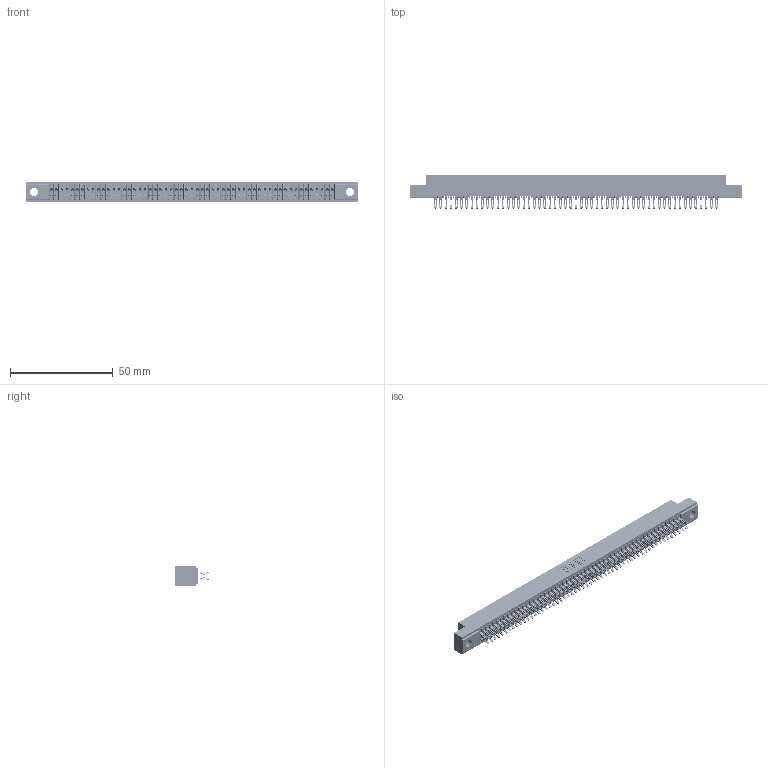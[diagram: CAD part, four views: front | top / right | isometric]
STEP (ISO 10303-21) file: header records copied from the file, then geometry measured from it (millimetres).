
FILE_DESCRIPTION (( 'STEP AP203' ), '1' );
FILE_NAME ('391-110-555-204.STEP', '2018-08-09T21:50:41', ( '' ), ( '' ), 'SwSTEP 2.0', 'SolidWorks 2016', '' );
FILE_SCHEMA (( 'CONFIG_CONTROL_DESIGN' ));
Length unit declared in the file: inch
Products named in the file (3): 341 Part_.156 (3.96) Dia Mounting Holes; 341-292-001_341-292-155; 391-110-555-204
Assembly tree (111 placements, depth 2):
  391-110-555-204
    341 Part_.156 (3.96) Dia Mounting Holes
    341-292-001_341-292-155  x110
Bounding box: 161.93 x 16.31 x 10.16 mm (x, y, z)
Volume: 12002.7 mm3; surface area: 22500.8 mm2
Topology: 111 solids, 111 shells, 8710 faces, 26037 edges, 16950 vertices
Faces by surface type: plane 4702, cylinder 3788, sphere 112, torus 108
Entity records: 65718 total; most frequent: CARTESIAN_POINT 10945, ORIENTED_EDGE 10866, DIRECTION 10595, EDGE_CURVE 5433, LINE 4395, VECTOR 4395, VERTEX_POINT 3434, AXIS2_PLACEMENT_3D 3100
